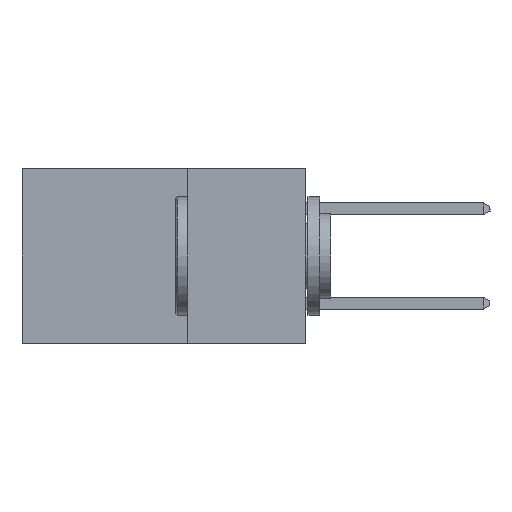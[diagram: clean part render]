
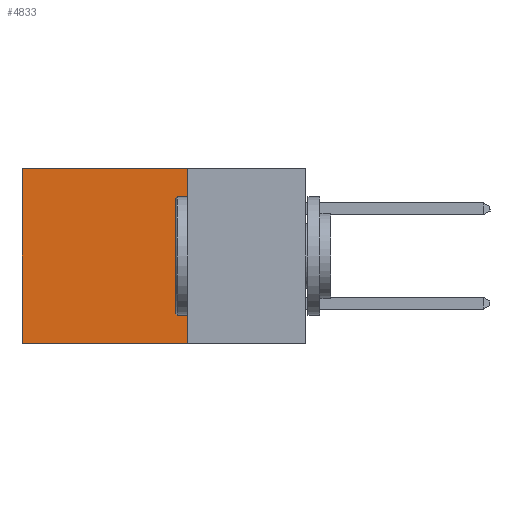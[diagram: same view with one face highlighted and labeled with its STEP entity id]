
A CAD part, left-side view. The second image highlights one B-rep face of the part: STEP entity #4833.
In plain terms, the highlighted planar face has unit normal (-1, 0, 0).
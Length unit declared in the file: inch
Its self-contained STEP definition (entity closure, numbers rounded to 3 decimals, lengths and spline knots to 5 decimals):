
#1061 = ORIENTED_EDGE ( 'NONE', *, *, #2017, .F. ) ;
#1064 = ORIENTED_EDGE ( 'NONE', *, *, #6176, .F. ) ;
#1374 = CARTESIAN_POINT ( 'NONE',  ( 0.298, 0.6, -0.37 ) ) ;
#2001 = VERTEX_POINT ( 'NONE', #5488 ) ;
#2017 = EDGE_CURVE ( 'NONE', #2001, #9496, #24938, .T. ) ;
#2242 = CARTESIAN_POINT ( 'NONE',  ( 0.298, 0.25, 0. ) ) ;
#4394 = EDGE_LOOP ( 'NONE', ( #9244, #1061, #1064, #14777 ) ) ;
#4833 = ADVANCED_FACE ( 'NONE', ( #20054 ), #23789, .F. ) ;
#4976 = VECTOR ( 'NONE', #14492, 39.37008 ) ;
#5488 = CARTESIAN_POINT ( 'NONE',  ( 0.298, 0.25, -0.37 ) ) ;
#6176 = EDGE_CURVE ( 'NONE', #6440, #2001, #18672, .T. ) ;
#6440 = VERTEX_POINT ( 'NONE', #23433 ) ;
#6885 = VECTOR ( 'NONE', #12669, 39.37008 ) ;
#7199 = DIRECTION ( 'NONE',  ( 0., 1., 0. ) ) ;
#8768 = CARTESIAN_POINT ( 'NONE',  ( 0.298, 0.25, 0. ) ) ;
#9244 = ORIENTED_EDGE ( 'NONE', *, *, #17384, .T. ) ;
#9496 = VERTEX_POINT ( 'NONE', #1374 ) ;
#10854 = CARTESIAN_POINT ( 'NONE',  ( 0.298, 0.6, 0. ) ) ;
#11389 = AXIS2_PLACEMENT_3D ( 'NONE', #8768, #19217, #19748 ) ;
#11751 = CARTESIAN_POINT ( 'NONE',  ( 0.298, 0.6, 0. ) ) ;
#12669 = DIRECTION ( 'NONE',  ( 0., 0., -1. ) ) ;
#13961 = VECTOR ( 'NONE', #7199, 39.37008 ) ;
#14492 = DIRECTION ( 'NONE',  ( 0., 1., 0. ) ) ;
#14777 = ORIENTED_EDGE ( 'NONE', *, *, #23257, .T. ) ;
#17164 = VECTOR ( 'NONE', #18055, 39.37008 ) ;
#17384 = EDGE_CURVE ( 'NONE', #18766, #9496, #22640, .T. ) ;
#18055 = DIRECTION ( 'NONE',  ( 0., 0., -1. ) ) ;
#18672 = LINE ( 'NONE', #2242, #6885 ) ;
#18766 = VERTEX_POINT ( 'NONE', #10854 ) ;
#19217 = DIRECTION ( 'NONE',  ( 1., 0., 0. ) ) ;
#19748 = DIRECTION ( 'NONE',  ( 0., 0., -1. ) ) ;
#20054 = FACE_OUTER_BOUND ( 'NONE', #4394, .T. ) ;
#20955 = LINE ( 'NONE', #24764, #4976 ) ;
#21992 = CARTESIAN_POINT ( 'NONE',  ( 0.298, 0.25, -0.37 ) ) ;
#22640 = LINE ( 'NONE', #11751, #17164 ) ;
#23257 = EDGE_CURVE ( 'NONE', #6440, #18766, #20955, .T. ) ;
#23433 = CARTESIAN_POINT ( 'NONE',  ( 0.298, 0.25, 0. ) ) ;
#23789 = PLANE ( 'NONE',  #11389 ) ;
#24764 = CARTESIAN_POINT ( 'NONE',  ( 0.298, 0.25, 0. ) ) ;
#24938 = LINE ( 'NONE', #21992, #13961 ) ;
